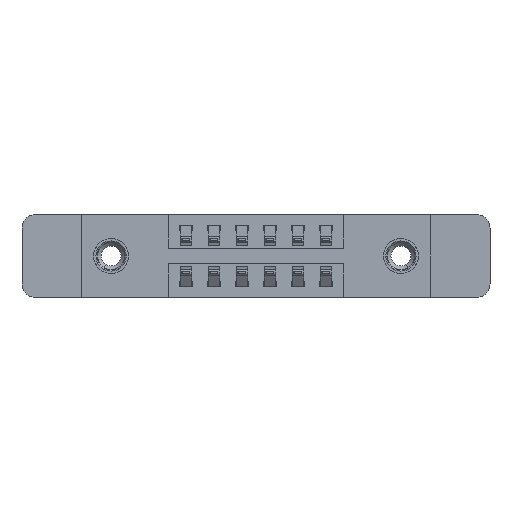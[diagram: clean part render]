
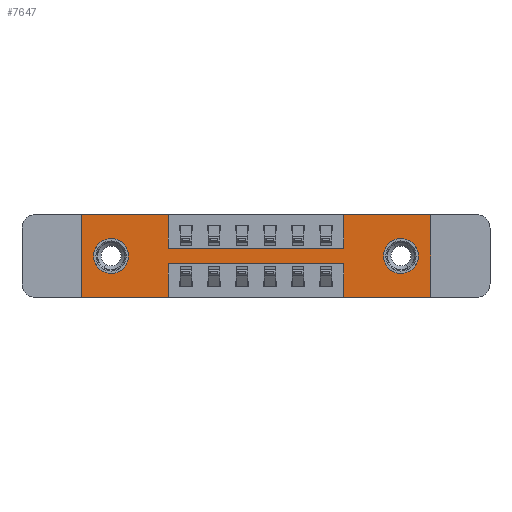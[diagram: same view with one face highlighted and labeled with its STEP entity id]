
A CAD part, front view. The second image highlights one B-rep face of the part: STEP entity #7647.
In plain terms, the highlighted planar face has unit normal (0, -1, 0).
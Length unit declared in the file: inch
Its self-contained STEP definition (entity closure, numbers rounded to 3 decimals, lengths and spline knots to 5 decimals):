
#137 = DIRECTION ( 'NONE',  ( 0., 1., 0. ) ) ;
#147 = ORIENTED_EDGE ( 'NONE', *, *, #1321, .F. ) ;
#278 = CARTESIAN_POINT ( 'NONE',  ( 1.1725, 0., -0.15 ) ) ;
#316 = EDGE_CURVE ( 'NONE', #6281, #11277, #605, .T. ) ;
#504 = ORIENTED_EDGE ( 'NONE', *, *, #7597, .T. ) ;
#605 = LINE ( 'NONE', #5608, #6024 ) ;
#629 = LINE ( 'NONE', #11560, #13037 ) ;
#695 = EDGE_CURVE ( 'NONE', #12882, #5415, #8652, .T. ) ;
#830 = ORIENTED_EDGE ( 'NONE', *, *, #9935, .F. ) ;
#844 = DIRECTION ( 'NONE',  ( 0., 0., 1. ) ) ;
#848 = LINE ( 'NONE', #11990, #9171 ) ;
#1069 = DIRECTION ( 'NONE',  ( 0., 0., -1. ) ) ;
#1085 = DIRECTION ( 'NONE',  ( 0., 0., 1. ) ) ;
#1281 = VECTOR ( 'NONE', #1069, 39.37008 ) ;
#1321 = EDGE_CURVE ( 'NONE', #11277, #12882, #629, .T. ) ;
#1333 = FACE_BOUND ( 'NONE', #12432, .T. ) ;
#1536 = CIRCLE ( 'NONE', #10059, 0.078 ) ;
#1623 = CARTESIAN_POINT ( 'NONE',  ( 1.56, 0., 0. ) ) ;
#1639 = CARTESIAN_POINT ( 'NONE',  ( 0.3875, 0., -0.15 ) ) ;
#1656 = FACE_OUTER_BOUND ( 'NONE', #2054, .T. ) ;
#1959 = CARTESIAN_POINT ( 'NONE',  ( 1.56, 0., -0.37 ) ) ;
#1962 = CARTESIAN_POINT ( 'NONE',  ( 0.3875, 0., -0.22 ) ) ;
#2054 = EDGE_LOOP ( 'NONE', ( #2586, #5779, #147, #11807, #6837, #9459, #11036, #5284, #2570, #830, #13604, #7981 ) ) ;
#2129 = CARTESIAN_POINT ( 'NONE',  ( 1.1725, 0., 0. ) ) ;
#2271 = DIRECTION ( 'NONE',  ( 0., 0., -1. ) ) ;
#2328 = EDGE_CURVE ( 'NONE', #10518, #10316, #8606, .T. ) ;
#2339 = CARTESIAN_POINT ( 'NONE',  ( 0., 0., -0.37 ) ) ;
#2570 = ORIENTED_EDGE ( 'NONE', *, *, #8974, .F. ) ;
#2586 = ORIENTED_EDGE ( 'NONE', *, *, #7836, .F. ) ;
#3032 = VERTEX_POINT ( 'NONE', #7450 ) ;
#3033 = DIRECTION ( 'NONE',  ( 0., 1., 0. ) ) ;
#3265 = DIRECTION ( 'NONE',  ( -1., 0., 0. ) ) ;
#3780 = DIRECTION ( 'NONE',  ( 0., 0., -1. ) ) ;
#3834 = AXIS2_PLACEMENT_3D ( 'NONE', #12552, #10284, #3780 ) ;
#3922 = DIRECTION ( 'NONE',  ( 0., 1., 0. ) ) ;
#3937 = DIRECTION ( 'NONE',  ( 0., 0., 1. ) ) ;
#3968 = CIRCLE ( 'NONE', #10345, 0.078 ) ;
#4029 = EDGE_CURVE ( 'NONE', #12413, #11470, #3968, .T. ) ;
#4179 = CARTESIAN_POINT ( 'NONE',  ( 0.1325, 0., -0.185 ) ) ;
#4356 = VECTOR ( 'NONE', #7922, 39.37008 ) ;
#4628 = EDGE_CURVE ( 'NONE', #12058, #6281, #13613, .T. ) ;
#4695 = DIRECTION ( 'NONE',  ( -1., 0., 0. ) ) ;
#5284 = ORIENTED_EDGE ( 'NONE', *, *, #2328, .F. ) ;
#5383 = FACE_BOUND ( 'NONE', #13854, .T. ) ;
#5390 = CARTESIAN_POINT ( 'NONE',  ( 0., 0., 0. ) ) ;
#5398 = DIRECTION ( 'NONE',  ( 1., 0., 0. ) ) ;
#5415 = VERTEX_POINT ( 'NONE', #12197 ) ;
#5608 = CARTESIAN_POINT ( 'NONE',  ( 0., 0., -0.37 ) ) ;
#5752 = VECTOR ( 'NONE', #3265, 39.37008 ) ;
#5770 = ORIENTED_EDGE ( 'NONE', *, *, #12242, .T. ) ;
#5779 = ORIENTED_EDGE ( 'NONE', *, *, #695, .F. ) ;
#5836 = CARTESIAN_POINT ( 'NONE',  ( 1.56, 0., 0. ) ) ;
#5854 = EDGE_CURVE ( 'NONE', #13003, #10106, #10880, .T. ) ;
#5886 = EDGE_CURVE ( 'NONE', #13144, #13003, #848, .T. ) ;
#5893 = CARTESIAN_POINT ( 'NONE',  ( 0.3875, 0., -0.15 ) ) ;
#5918 = CARTESIAN_POINT ( 'NONE',  ( 0.1325, 0., -0.107 ) ) ;
#6024 = VECTOR ( 'NONE', #4695, 39.37008 ) ;
#6139 = CARTESIAN_POINT ( 'NONE',  ( 0.3875, 0., 0. ) ) ;
#6281 = VERTEX_POINT ( 'NONE', #1959 ) ;
#6477 = DIRECTION ( 'NONE',  ( -1., 0., 0. ) ) ;
#6732 = AXIS2_PLACEMENT_3D ( 'NONE', #4179, #7383, #844 ) ;
#6748 = CIRCLE ( 'NONE', #11840, 0.078 ) ;
#6837 = ORIENTED_EDGE ( 'NONE', *, *, #4628, .F. ) ;
#6886 = LINE ( 'NONE', #6139, #11476 ) ;
#6896 = LINE ( 'NONE', #11886, #1281 ) ;
#7171 = VERTEX_POINT ( 'NONE', #5918 ) ;
#7274 = CIRCLE ( 'NONE', #6732, 0.078 ) ;
#7310 = CARTESIAN_POINT ( 'NONE',  ( 0.1325, 0., -0.263 ) ) ;
#7371 = EDGE_CURVE ( 'NONE', #12592, #12058, #11853, .T. ) ;
#7383 = DIRECTION ( 'NONE',  ( 0., 1., 0. ) ) ;
#7450 = CARTESIAN_POINT ( 'NONE',  ( 0.3875, 0., 0. ) ) ;
#7483 = CARTESIAN_POINT ( 'NONE',  ( 0., 0., 0. ) ) ;
#7485 = VECTOR ( 'NONE', #8575, 39.37008 ) ;
#7597 = EDGE_CURVE ( 'NONE', #7171, #11329, #6748, .T. ) ;
#7647 = ADVANCED_FACE ( 'NONE', ( #1333, #5383, #1656 ), #9180, .T. ) ;
#7836 = EDGE_CURVE ( 'NONE', #5415, #13144, #6896, .T. ) ;
#7922 = DIRECTION ( 'NONE',  ( 1., 0., 0. ) ) ;
#7981 = ORIENTED_EDGE ( 'NONE', *, *, #5886, .F. ) ;
#8422 = CARTESIAN_POINT ( 'NONE',  ( 1.4275, 0., -0.185 ) ) ;
#8471 = DIRECTION ( 'NONE',  ( 0., 0., -1. ) ) ;
#8575 = DIRECTION ( 'NONE',  ( 0., 0., 1. ) ) ;
#8606 = LINE ( 'NONE', #5893, #4356 ) ;
#8652 = LINE ( 'NONE', #1962, #5752 ) ;
#8676 = CARTESIAN_POINT ( 'NONE',  ( 1.4275, 0., -0.263 ) ) ;
#8723 = CARTESIAN_POINT ( 'NONE',  ( 0., 0., 0. ) ) ;
#8815 = DIRECTION ( 'NONE',  ( 1., 0., 0. ) ) ;
#8974 = EDGE_CURVE ( 'NONE', #3032, #10518, #6886, .T. ) ;
#9171 = VECTOR ( 'NONE', #6477, 39.37008 ) ;
#9180 = PLANE ( 'NONE',  #3834 ) ;
#9459 = ORIENTED_EDGE ( 'NONE', *, *, #7371, .F. ) ;
#9533 = CARTESIAN_POINT ( 'NONE',  ( 1.1725, 0., -0.37 ) ) ;
#9563 = VECTOR ( 'NONE', #5398, 39.37008 ) ;
#9636 = VECTOR ( 'NONE', #8815, 39.37008 ) ;
#9935 = EDGE_CURVE ( 'NONE', #10106, #3032, #12819, .T. ) ;
#10004 = CARTESIAN_POINT ( 'NONE',  ( 1.1725, 0., 0. ) ) ;
#10059 = AXIS2_PLACEMENT_3D ( 'NONE', #8422, #3033, #8471 ) ;
#10106 = VERTEX_POINT ( 'NONE', #14020 ) ;
#10284 = DIRECTION ( 'NONE',  ( 0., -1., 0. ) ) ;
#10316 = VERTEX_POINT ( 'NONE', #278 ) ;
#10345 = AXIS2_PLACEMENT_3D ( 'NONE', #13147, #137, #2271 ) ;
#10372 = ORIENTED_EDGE ( 'NONE', *, *, #13953, .T. ) ;
#10518 = VERTEX_POINT ( 'NONE', #1639 ) ;
#10710 = CARTESIAN_POINT ( 'NONE',  ( 1.1725, 0., -0.22 ) ) ;
#10880 = LINE ( 'NONE', #5390, #12404 ) ;
#10882 = CARTESIAN_POINT ( 'NONE',  ( 1.4275, 0., -0.107 ) ) ;
#11036 = ORIENTED_EDGE ( 'NONE', *, *, #12218, .F. ) ;
#11277 = VERTEX_POINT ( 'NONE', #9533 ) ;
#11329 = VERTEX_POINT ( 'NONE', #7310 ) ;
#11470 = VERTEX_POINT ( 'NONE', #10882 ) ;
#11476 = VECTOR ( 'NONE', #12760, 39.37008 ) ;
#11560 = CARTESIAN_POINT ( 'NONE',  ( 1.1725, 0., -0.37 ) ) ;
#11807 = ORIENTED_EDGE ( 'NONE', *, *, #316, .F. ) ;
#11840 = AXIS2_PLACEMENT_3D ( 'NONE', #13490, #3922, #12458 ) ;
#11853 = LINE ( 'NONE', #8723, #9636 ) ;
#11886 = CARTESIAN_POINT ( 'NONE',  ( 0.3875, 0., -0.37 ) ) ;
#11990 = CARTESIAN_POINT ( 'NONE',  ( 0., 0., -0.37 ) ) ;
#12058 = VERTEX_POINT ( 'NONE', #5836 ) ;
#12197 = CARTESIAN_POINT ( 'NONE',  ( 0.3875, 0., -0.22 ) ) ;
#12218 = EDGE_CURVE ( 'NONE', #10316, #12592, #13264, .T. ) ;
#12242 = EDGE_CURVE ( 'NONE', #11470, #12413, #1536, .T. ) ;
#12404 = VECTOR ( 'NONE', #1085, 39.37008 ) ;
#12406 = ORIENTED_EDGE ( 'NONE', *, *, #4029, .T. ) ;
#12413 = VERTEX_POINT ( 'NONE', #8676 ) ;
#12432 = EDGE_LOOP ( 'NONE', ( #5770, #12406 ) ) ;
#12441 = VECTOR ( 'NONE', #12496, 39.37008 ) ;
#12458 = DIRECTION ( 'NONE',  ( 0., 0., 1. ) ) ;
#12496 = DIRECTION ( 'NONE',  ( 0., 0., -1. ) ) ;
#12552 = CARTESIAN_POINT ( 'NONE',  ( 0., 0., -0.37 ) ) ;
#12592 = VERTEX_POINT ( 'NONE', #10004 ) ;
#12760 = DIRECTION ( 'NONE',  ( 0., 0., -1. ) ) ;
#12819 = LINE ( 'NONE', #7483, #9563 ) ;
#12882 = VERTEX_POINT ( 'NONE', #10710 ) ;
#13003 = VERTEX_POINT ( 'NONE', #2339 ) ;
#13037 = VECTOR ( 'NONE', #3937, 39.37008 ) ;
#13144 = VERTEX_POINT ( 'NONE', #13479 ) ;
#13147 = CARTESIAN_POINT ( 'NONE',  ( 1.4275, 0., -0.185 ) ) ;
#13264 = LINE ( 'NONE', #2129, #7485 ) ;
#13479 = CARTESIAN_POINT ( 'NONE',  ( 0.3875, 0., -0.37 ) ) ;
#13490 = CARTESIAN_POINT ( 'NONE',  ( 0.1325, 0., -0.185 ) ) ;
#13604 = ORIENTED_EDGE ( 'NONE', *, *, #5854, .F. ) ;
#13613 = LINE ( 'NONE', #1623, #12441 ) ;
#13854 = EDGE_LOOP ( 'NONE', ( #504, #10372 ) ) ;
#13953 = EDGE_CURVE ( 'NONE', #11329, #7171, #7274, .T. ) ;
#14020 = CARTESIAN_POINT ( 'NONE',  ( 0., 0., 0. ) ) ;
